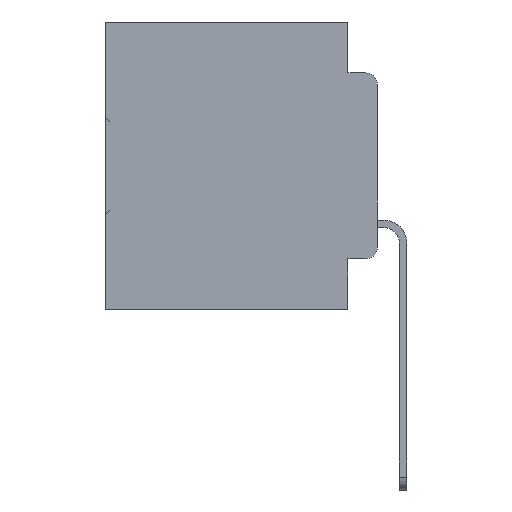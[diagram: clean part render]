
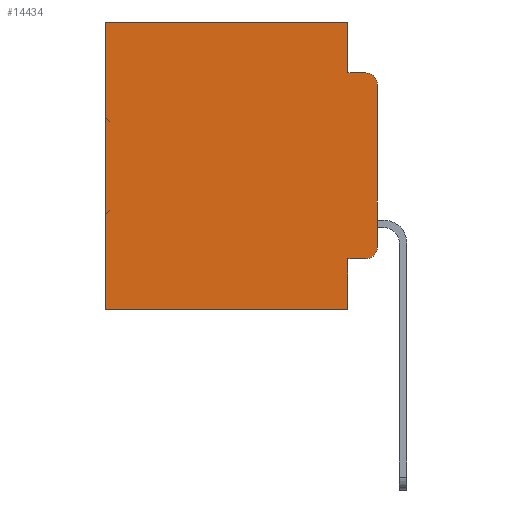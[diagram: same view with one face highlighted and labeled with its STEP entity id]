
A CAD part, left-side view. The second image highlights one B-rep face of the part: STEP entity #14434.
In plain terms, the highlighted planar face has unit normal (-1, 0, 0).
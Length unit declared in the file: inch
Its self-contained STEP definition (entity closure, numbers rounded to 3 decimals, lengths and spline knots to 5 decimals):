
#271 = LINE ( 'NONE', #34003, #36602 ) ;
#273 = ORIENTED_EDGE ( 'NONE', *, *, #14673, .T. ) ;
#1035 = EDGE_CURVE ( 'NONE', #22932, #19335, #37028, .T. ) ;
#1857 = CARTESIAN_POINT ( 'NONE',  ( 0.298, 0., 0. ) ) ;
#3230 = VECTOR ( 'NONE', #6853, 39.37008 ) ;
#3732 = LINE ( 'NONE', #33728, #10658 ) ;
#4726 = LINE ( 'NONE', #5060, #12493 ) ;
#4918 = DIRECTION ( 'NONE',  ( 0., 0., -1. ) ) ;
#4948 = CIRCLE ( 'NONE', #10323, 0.02 ) ;
#5060 = CARTESIAN_POINT ( 'NONE',  ( 0.298, 0., 0. ) ) ;
#5438 = CARTESIAN_POINT ( 'NONE',  ( 0.298, 0.473, -0.5 ) ) ;
#5721 = ORIENTED_EDGE ( 'NONE', *, *, #21406, .T. ) ;
#6747 = CARTESIAN_POINT ( 'NONE',  ( 0.298, 0.051, 0. ) ) ;
#6846 = DIRECTION ( 'NONE',  ( 0., 0., -1. ) ) ;
#6853 = DIRECTION ( 'NONE',  ( 0., 0., -1. ) ) ;
#8408 = DIRECTION ( 'NONE',  ( -1., 0., 0. ) ) ;
#8757 = DIRECTION ( 'NONE',  ( -1., 0., 0. ) ) ;
#9573 = EDGE_LOOP ( 'NONE', ( #29687, #17293, #19110, #28439, #273, #15966, #18278, #17481, #35096, #5721 ) ) ;
#9802 = CARTESIAN_POINT ( 'NONE',  ( 0.298, 0.02, -0.0885 ) ) ;
#10323 = AXIS2_PLACEMENT_3D ( 'NONE', #25956, #8757, #28806 ) ;
#10658 = VECTOR ( 'NONE', #25307, 39.37008 ) ;
#10867 = VERTEX_POINT ( 'NONE', #13419 ) ;
#10872 = VERTEX_POINT ( 'NONE', #22013 ) ;
#11960 = DIRECTION ( 'NONE',  ( 0., 0., -1. ) ) ;
#12493 = VECTOR ( 'NONE', #30775, 39.37008 ) ;
#13265 = VERTEX_POINT ( 'NONE', #6747 ) ;
#13419 = CARTESIAN_POINT ( 'NONE',  ( 0.298, 0.02, -0.4115 ) ) ;
#13661 = VERTEX_POINT ( 'NONE', #28480 ) ;
#14365 = VERTEX_POINT ( 'NONE', #34856 ) ;
#14434 = ADVANCED_FACE ( 'NONE', ( #34655 ), #24143, .F. ) ;
#14673 = EDGE_CURVE ( 'NONE', #13265, #22932, #4726, .T. ) ;
#15151 = VECTOR ( 'NONE', #24432, 39.37008 ) ;
#15495 = DIRECTION ( 'NONE',  ( 1., 0., 0. ) ) ;
#15966 = ORIENTED_EDGE ( 'NONE', *, *, #1035, .T. ) ;
#16082 = EDGE_CURVE ( 'NONE', #14365, #30041, #4948, .T. ) ;
#16845 = DIRECTION ( 'NONE',  ( 0., -1., 0. ) ) ;
#17293 = ORIENTED_EDGE ( 'NONE', *, *, #16082, .T. ) ;
#17311 = AXIS2_PLACEMENT_3D ( 'NONE', #21333, #15495, #6846 ) ;
#17481 = ORIENTED_EDGE ( 'NONE', *, *, #34491, .F. ) ;
#18278 = ORIENTED_EDGE ( 'NONE', *, *, #29673, .F. ) ;
#18749 = CARTESIAN_POINT ( 'NONE',  ( 0.298, 0.051, -0.0885 ) ) ;
#18758 = EDGE_CURVE ( 'NONE', #13265, #34777, #33695, .T. ) ;
#19110 = ORIENTED_EDGE ( 'NONE', *, *, #28247, .F. ) ;
#19253 = EDGE_CURVE ( 'NONE', #14365, #10872, #22762, .T. ) ;
#19335 = VERTEX_POINT ( 'NONE', #5438 ) ;
#21176 = CARTESIAN_POINT ( 'NONE',  ( 0.298, 0.473, 0. ) ) ;
#21333 = CARTESIAN_POINT ( 'NONE',  ( 0.298, 0., 0. ) ) ;
#21406 = EDGE_CURVE ( 'NONE', #10867, #10872, #33374, .T. ) ;
#22013 = CARTESIAN_POINT ( 'NONE',  ( 0.298, 0., -0.3915 ) ) ;
#22190 = CARTESIAN_POINT ( 'NONE',  ( 0.298, 0.051, -0.4115 ) ) ;
#22309 = VECTOR ( 'NONE', #16845, 39.37008 ) ;
#22762 = LINE ( 'NONE', #1857, #36637 ) ;
#22932 = VERTEX_POINT ( 'NONE', #21176 ) ;
#23314 = EDGE_CURVE ( 'NONE', #33598, #10867, #36210, .T. ) ;
#23422 = CARTESIAN_POINT ( 'NONE',  ( 0.298, 0.473, 0. ) ) ;
#24143 = PLANE ( 'NONE',  #17311 ) ;
#24152 = CARTESIAN_POINT ( 'NONE',  ( 0.298, 0.051, 0. ) ) ;
#24432 = DIRECTION ( 'NONE',  ( 0., -1., 0. ) ) ;
#24551 = LINE ( 'NONE', #18749, #15151 ) ;
#25307 = DIRECTION ( 'NONE',  ( 0., 0., -1. ) ) ;
#25612 = CARTESIAN_POINT ( 'NONE',  ( 0.298, 0.02, -0.3915 ) ) ;
#25956 = CARTESIAN_POINT ( 'NONE',  ( 0.298, 0.02, -0.1085 ) ) ;
#28174 = CARTESIAN_POINT ( 'NONE',  ( 0.298, 0.051, -0.4115 ) ) ;
#28247 = EDGE_CURVE ( 'NONE', #34777, #30041, #24551, .T. ) ;
#28439 = ORIENTED_EDGE ( 'NONE', *, *, #18758, .F. ) ;
#28467 = DIRECTION ( 'NONE',  ( 0., 0., -1. ) ) ;
#28480 = CARTESIAN_POINT ( 'NONE',  ( 0.298, 0.051, -0.5 ) ) ;
#28806 = DIRECTION ( 'NONE',  ( 0., 0., -1. ) ) ;
#29673 = EDGE_CURVE ( 'NONE', #13661, #19335, #271, .T. ) ;
#29687 = ORIENTED_EDGE ( 'NONE', *, *, #19253, .F. ) ;
#29738 = VECTOR ( 'NONE', #11960, 39.37008 ) ;
#30041 = VERTEX_POINT ( 'NONE', #9802 ) ;
#30146 = CARTESIAN_POINT ( 'NONE',  ( 0.298, 0.051, -0.0885 ) ) ;
#30775 = DIRECTION ( 'NONE',  ( 0., 1., 0. ) ) ;
#32628 = AXIS2_PLACEMENT_3D ( 'NONE', #25612, #8408, #28467 ) ;
#33374 = CIRCLE ( 'NONE', #32628, 0.02 ) ;
#33598 = VERTEX_POINT ( 'NONE', #22190 ) ;
#33695 = LINE ( 'NONE', #24152, #3230 ) ;
#33728 = CARTESIAN_POINT ( 'NONE',  ( 0.298, 0.051, 0. ) ) ;
#34003 = CARTESIAN_POINT ( 'NONE',  ( 0.298, 0., -0.5 ) ) ;
#34491 = EDGE_CURVE ( 'NONE', #33598, #13661, #3732, .T. ) ;
#34655 = FACE_OUTER_BOUND ( 'NONE', #9573, .T. ) ;
#34777 = VERTEX_POINT ( 'NONE', #30146 ) ;
#34856 = CARTESIAN_POINT ( 'NONE',  ( 0.298, 0., -0.1085 ) ) ;
#35096 = ORIENTED_EDGE ( 'NONE', *, *, #23314, .T. ) ;
#36210 = LINE ( 'NONE', #28174, #22309 ) ;
#36602 = VECTOR ( 'NONE', #36743, 39.37008 ) ;
#36637 = VECTOR ( 'NONE', #4918, 39.37008 ) ;
#36743 = DIRECTION ( 'NONE',  ( 0., 1., 0. ) ) ;
#37028 = LINE ( 'NONE', #23422, #29738 ) ;
